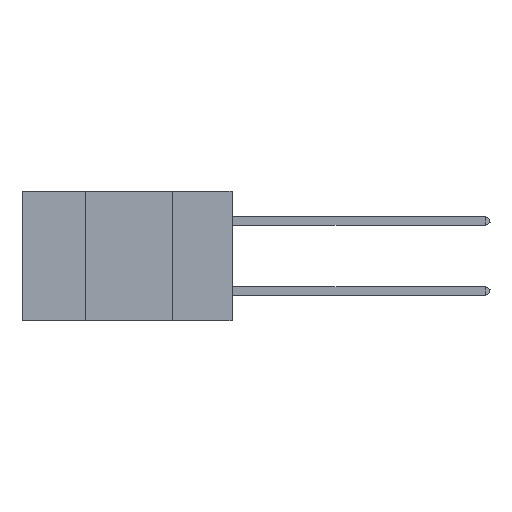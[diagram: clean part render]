
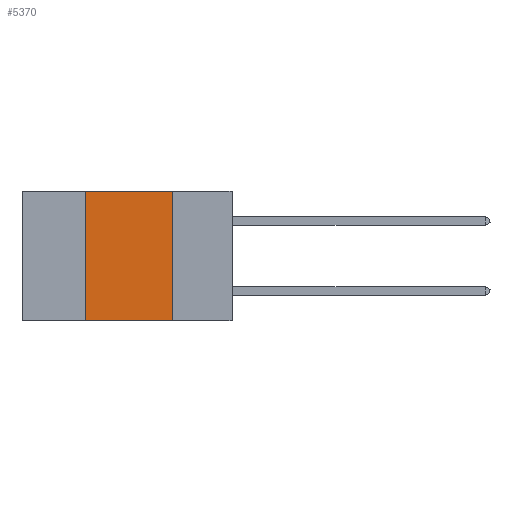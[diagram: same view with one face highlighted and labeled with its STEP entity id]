
A CAD part, left-side view. The second image highlights one B-rep face of the part: STEP entity #5370.
In plain terms, the highlighted planar face has unit normal (-1, 0, 0).
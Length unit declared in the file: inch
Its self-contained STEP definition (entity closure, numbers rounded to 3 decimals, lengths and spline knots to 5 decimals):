
#2029 = ORIENTED_EDGE ( 'NONE', *, *, #33469, .T. ) ;
#2471 = LINE ( 'NONE', #15257, #31464 ) ;
#3149 = VERTEX_POINT ( 'NONE', #33528 ) ;
#3505 = EDGE_CURVE ( 'NONE', #3149, #7541, #18455, .T. ) ;
#3771 = LINE ( 'NONE', #25462, #36040 ) ;
#5370 = ADVANCED_FACE ( 'NONE', ( #25420 ), #26913, .F. ) ;
#5481 = DIRECTION ( 'NONE',  ( 0., 0., -1. ) ) ;
#6776 = CARTESIAN_POINT ( 'NONE',  ( 0., 0.17, -0.37 ) ) ;
#7491 = ORIENTED_EDGE ( 'NONE', *, *, #22845, .F. ) ;
#7541 = VERTEX_POINT ( 'NONE', #6776 ) ;
#10549 = CARTESIAN_POINT ( 'NONE',  ( 0., 0.6, 0. ) ) ;
#11249 = VERTEX_POINT ( 'NONE', #36601 ) ;
#15257 = CARTESIAN_POINT ( 'NONE',  ( 0., 0.42, 0. ) ) ;
#17605 = VERTEX_POINT ( 'NONE', #25168 ) ;
#18455 = LINE ( 'NONE', #33404, #38305 ) ;
#19274 = EDGE_CURVE ( 'NONE', #11249, #17605, #2471, .T. ) ;
#19414 = DIRECTION ( 'NONE',  ( 0., -1., 0. ) ) ;
#22845 = EDGE_CURVE ( 'NONE', #17605, #3149, #34836, .T. ) ;
#23978 = DIRECTION ( 'NONE',  ( 1., 0., 0. ) ) ;
#24330 = DIRECTION ( 'NONE',  ( 0., 0., -1. ) ) ;
#25168 = CARTESIAN_POINT ( 'NONE',  ( 0., 0.42, 0. ) ) ;
#25420 = FACE_OUTER_BOUND ( 'NONE', #31339, .T. ) ;
#25462 = CARTESIAN_POINT ( 'NONE',  ( 0., 0.6, -0.37 ) ) ;
#25598 = DIRECTION ( 'NONE',  ( 0., -1., 0. ) ) ;
#26775 = CARTESIAN_POINT ( 'NONE',  ( 0., 0.6, 0. ) ) ;
#26913 = PLANE ( 'NONE',  #28705 ) ;
#28705 = AXIS2_PLACEMENT_3D ( 'NONE', #26775, #23978, #5481 ) ;
#31339 = EDGE_LOOP ( 'NONE', ( #38235, #7491, #33719, #2029 ) ) ;
#31464 = VECTOR ( 'NONE', #36450, 39.37008 ) ;
#31533 = VECTOR ( 'NONE', #19414, 39.37008 ) ;
#33404 = CARTESIAN_POINT ( 'NONE',  ( 0., 0.17, 0. ) ) ;
#33469 = EDGE_CURVE ( 'NONE', #11249, #7541, #3771, .T. ) ;
#33528 = CARTESIAN_POINT ( 'NONE',  ( 0., 0.17, 0. ) ) ;
#33719 = ORIENTED_EDGE ( 'NONE', *, *, #19274, .F. ) ;
#34836 = LINE ( 'NONE', #10549, #31533 ) ;
#36040 = VECTOR ( 'NONE', #25598, 39.37008 ) ;
#36450 = DIRECTION ( 'NONE',  ( 0., 0., 1. ) ) ;
#36601 = CARTESIAN_POINT ( 'NONE',  ( 0., 0.42, -0.37 ) ) ;
#38235 = ORIENTED_EDGE ( 'NONE', *, *, #3505, .F. ) ;
#38305 = VECTOR ( 'NONE', #24330, 39.37008 ) ;
